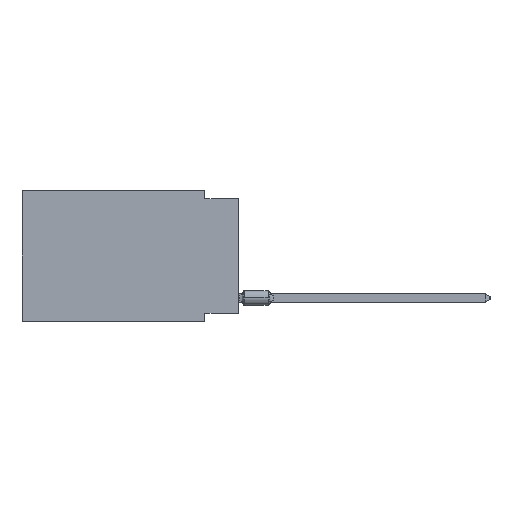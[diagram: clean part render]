
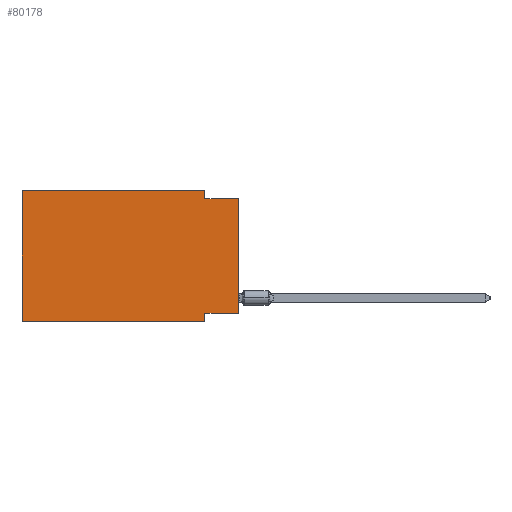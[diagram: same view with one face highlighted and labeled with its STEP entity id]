
A CAD part, left-side view. The second image highlights one B-rep face of the part: STEP entity #80178.
In plain terms, the highlighted planar face has unit normal (-1, 0, 0).
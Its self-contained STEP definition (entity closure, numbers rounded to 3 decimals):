
#23 = VERTEX_POINT ( 'NONE', #35757 ) ;
#641 = EDGE_LOOP ( 'NONE', ( #83551, #52529, #55176, #25912, #5770, #83496, #34202, #38209 ) ) ;
#898 = VECTOR ( 'NONE', #7502, 1000. ) ;
#1611 = VECTOR ( 'NONE', #64741, 1000. ) ;
#4094 = LINE ( 'NONE', #38863, #4131 ) ;
#4131 = VECTOR ( 'NONE', #72309, 1000. ) ;
#4147 = CARTESIAN_POINT ( 'NONE',  ( 0., 2.54, -0.635 ) ) ;
#4841 = EDGE_CURVE ( 'NONE', #5306, #31598, #70341, .T. ) ;
#5306 = VERTEX_POINT ( 'NONE', #85328 ) ;
#5770 = ORIENTED_EDGE ( 'NONE', *, *, #52634, .F. ) ;
#7502 = DIRECTION ( 'NONE',  ( 0., -1., 0. ) ) ;
#10008 = FACE_OUTER_BOUND ( 'NONE', #641, .T. ) ;
#10345 = CARTESIAN_POINT ( 'NONE',  ( 0., 16.383, 0. ) ) ;
#11740 = DIRECTION ( 'NONE',  ( 0., -1., 0. ) ) ;
#14611 = CARTESIAN_POINT ( 'NONE',  ( 0., 2.54, -9.271 ) ) ;
#17587 = DIRECTION ( 'NONE',  ( 0., 0., -1. ) ) ;
#18035 = DIRECTION ( 'NONE',  ( 1., 0., 0. ) ) ;
#18294 = LINE ( 'NONE', #53058, #21815 ) ;
#21815 = VECTOR ( 'NONE', #46796, 1000. ) ;
#23043 = VERTEX_POINT ( 'NONE', #4147 ) ;
#23813 = LINE ( 'NONE', #37185, #35570 ) ;
#25372 = VECTOR ( 'NONE', #86485, 1000. ) ;
#25440 = LINE ( 'NONE', #59329, #25372 ) ;
#25912 = ORIENTED_EDGE ( 'NONE', *, *, #4841, .F. ) ;
#27004 = VERTEX_POINT ( 'NONE', #31641 ) ;
#29957 = AXIS2_PLACEMENT_3D ( 'NONE', #31399, #18035, #17587 ) ;
#31399 = CARTESIAN_POINT ( 'NONE',  ( 0., 16.383, 0. ) ) ;
#31598 = VERTEX_POINT ( 'NONE', #73288 ) ;
#31641 = CARTESIAN_POINT ( 'NONE',  ( 0., 16.383, -9.906 ) ) ;
#34202 = ORIENTED_EDGE ( 'NONE', *, *, #36980, .F. ) ;
#34950 = EDGE_CURVE ( 'NONE', #31598, #23043, #61024, .T. ) ;
#35570 = VECTOR ( 'NONE', #63046, 1000. ) ;
#35757 = CARTESIAN_POINT ( 'NONE',  ( 0., 0., -9.271 ) ) ;
#36980 = EDGE_CURVE ( 'NONE', #74495, #66059, #18294, .T. ) ;
#37185 = CARTESIAN_POINT ( 'NONE',  ( 0., 0., -9.271 ) ) ;
#38209 = ORIENTED_EDGE ( 'NONE', *, *, #65250, .F. ) ;
#38863 = CARTESIAN_POINT ( 'NONE',  ( 0., 0., 0. ) ) ;
#39247 = CARTESIAN_POINT ( 'NONE',  ( 0., 2.54, 0. ) ) ;
#44230 = LINE ( 'NONE', #10345, #1611 ) ;
#46796 = DIRECTION ( 'NONE',  ( 0., 0., -1. ) ) ;
#50983 = LINE ( 'NONE', #58550, #65767 ) ;
#52336 = VECTOR ( 'NONE', #67295, 1000. ) ;
#52529 = ORIENTED_EDGE ( 'NONE', *, *, #68945, .F. ) ;
#52634 = EDGE_CURVE ( 'NONE', #27004, #5306, #44230, .T. ) ;
#53058 = CARTESIAN_POINT ( 'NONE',  ( 0., 2.54, -9.906 ) ) ;
#55176 = ORIENTED_EDGE ( 'NONE', *, *, #34950, .F. ) ;
#58550 = CARTESIAN_POINT ( 'NONE',  ( 0., 0., -0.635 ) ) ;
#59039 = PLANE ( 'NONE',  #29957 ) ;
#59166 = CARTESIAN_POINT ( 'NONE',  ( 0., 0., -0.635 ) ) ;
#59329 = CARTESIAN_POINT ( 'NONE',  ( 0., 16.383, -9.906 ) ) ;
#60956 = EDGE_CURVE ( 'NONE', #27004, #66059, #25440, .T. ) ;
#61024 = LINE ( 'NONE', #39247, #52336 ) ;
#63046 = DIRECTION ( 'NONE',  ( 0., 1., 0. ) ) ;
#64741 = DIRECTION ( 'NONE',  ( 0., 0., 1. ) ) ;
#65250 = EDGE_CURVE ( 'NONE', #23, #74495, #23813, .T. ) ;
#65767 = VECTOR ( 'NONE', #11740, 1000. ) ;
#66059 = VERTEX_POINT ( 'NONE', #67513 ) ;
#67295 = DIRECTION ( 'NONE',  ( 0., 0., -1. ) ) ;
#67513 = CARTESIAN_POINT ( 'NONE',  ( 0., 2.54, -9.906 ) ) ;
#68945 = EDGE_CURVE ( 'NONE', #23043, #70163, #50983, .T. ) ;
#70163 = VERTEX_POINT ( 'NONE', #59166 ) ;
#70341 = LINE ( 'NONE', #84125, #898 ) ;
#72309 = DIRECTION ( 'NONE',  ( 0., 0., 1. ) ) ;
#73288 = CARTESIAN_POINT ( 'NONE',  ( 0., 2.54, 0. ) ) ;
#74495 = VERTEX_POINT ( 'NONE', #14611 ) ;
#78982 = EDGE_CURVE ( 'NONE', #23, #70163, #4094, .T. ) ;
#80178 = ADVANCED_FACE ( 'NONE', ( #10008 ), #59039, .F. ) ;
#83496 = ORIENTED_EDGE ( 'NONE', *, *, #60956, .T. ) ;
#83551 = ORIENTED_EDGE ( 'NONE', *, *, #78982, .T. ) ;
#84125 = CARTESIAN_POINT ( 'NONE',  ( 0., 16.383, 0. ) ) ;
#85328 = CARTESIAN_POINT ( 'NONE',  ( 0., 16.383, 0. ) ) ;
#86485 = DIRECTION ( 'NONE',  ( 0., -1., 0. ) ) ;
